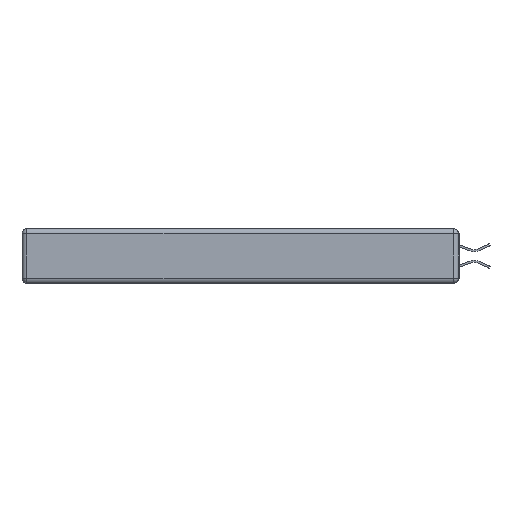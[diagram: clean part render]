
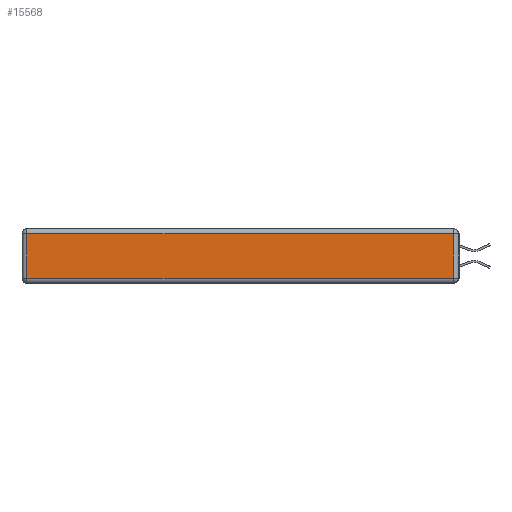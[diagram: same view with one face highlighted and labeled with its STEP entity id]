
A CAD part, left-side view. The second image highlights one B-rep face of the part: STEP entity #15568.
In plain terms, the highlighted planar face has unit normal (-1, 0, 0).
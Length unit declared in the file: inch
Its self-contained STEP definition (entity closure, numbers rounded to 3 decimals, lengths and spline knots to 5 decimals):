
#297 = EDGE_CURVE ( 'NONE', #7893, #11096, #5812, .T. ) ;
#793 = CARTESIAN_POINT ( 'NONE',  ( 0., 2.72, -0.03 ) ) ;
#967 = DIRECTION ( 'NONE',  ( 0., 0., -1. ) ) ;
#1071 = LINE ( 'NONE', #5270, #9946 ) ;
#1939 = DIRECTION ( 'NONE',  ( -1., 0., 0. ) ) ;
#2075 = EDGE_CURVE ( 'NONE', #4587, #15737, #16277, .T. ) ;
#3056 = CARTESIAN_POINT ( 'NONE',  ( 0., 0., -0.343 ) ) ;
#3323 = EDGE_LOOP ( 'NONE', ( #12599, #12824, #6045, #13713 ) ) ;
#4362 = EDGE_CURVE ( 'NONE', #15737, #7893, #8277, .T. ) ;
#4587 = VERTEX_POINT ( 'NONE', #793 ) ;
#5270 = CARTESIAN_POINT ( 'NONE',  ( 0., 2.75, -0.03 ) ) ;
#5812 = LINE ( 'NONE', #12532, #15735 ) ;
#6045 = ORIENTED_EDGE ( 'NONE', *, *, #10884, .T. ) ;
#6474 = VECTOR ( 'NONE', #13477, 39.37008 ) ;
#7011 = PLANE ( 'NONE',  #15223 ) ;
#7062 = CARTESIAN_POINT ( 'NONE',  ( 0., 0., -0.313 ) ) ;
#7870 = CARTESIAN_POINT ( 'NONE',  ( 0., 0.03, -0.313 ) ) ;
#7893 = VERTEX_POINT ( 'NONE', #7870 ) ;
#8277 = LINE ( 'NONE', #7062, #6474 ) ;
#9363 = CARTESIAN_POINT ( 'NONE',  ( 0., 0.03, -0.03 ) ) ;
#9946 = VECTOR ( 'NONE', #13182, 39.37008 ) ;
#10884 = EDGE_CURVE ( 'NONE', #11096, #4587, #1071, .T. ) ;
#10939 = CARTESIAN_POINT ( 'NONE',  ( 0., 2.72, -0.313 ) ) ;
#11096 = VERTEX_POINT ( 'NONE', #9363 ) ;
#12532 = CARTESIAN_POINT ( 'NONE',  ( 0., 0.03, -0.343 ) ) ;
#12599 = ORIENTED_EDGE ( 'NONE', *, *, #4362, .T. ) ;
#12824 = ORIENTED_EDGE ( 'NONE', *, *, #297, .T. ) ;
#13182 = DIRECTION ( 'NONE',  ( 0., 1., 0. ) ) ;
#13427 = DIRECTION ( 'NONE',  ( 0., 0., 1. ) ) ;
#13477 = DIRECTION ( 'NONE',  ( 0., -1., 0. ) ) ;
#13713 = ORIENTED_EDGE ( 'NONE', *, *, #2075, .T. ) ;
#14018 = VECTOR ( 'NONE', #967, 39.37008 ) ;
#14723 = FACE_OUTER_BOUND ( 'NONE', #3323, .T. ) ;
#15223 = AXIS2_PLACEMENT_3D ( 'NONE', #3056, #1939, #13427 ) ;
#15568 = ADVANCED_FACE ( 'NONE', ( #14723 ), #7011, .T. ) ;
#15735 = VECTOR ( 'NONE', #16346, 39.37008 ) ;
#15737 = VERTEX_POINT ( 'NONE', #10939 ) ;
#16277 = LINE ( 'NONE', #16752, #14018 ) ;
#16346 = DIRECTION ( 'NONE',  ( 0., 0., 1. ) ) ;
#16752 = CARTESIAN_POINT ( 'NONE',  ( 0., 2.72, -0.343 ) ) ;
